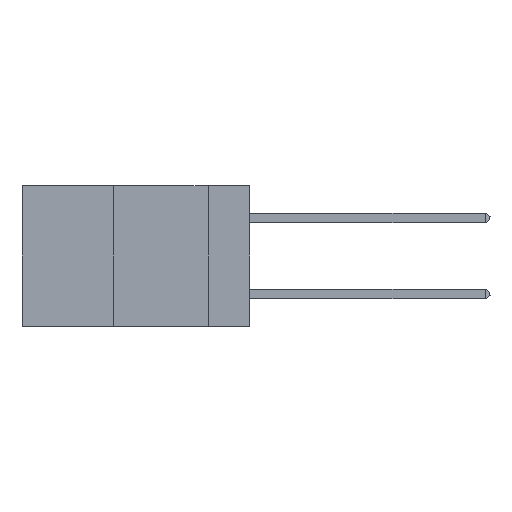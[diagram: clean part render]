
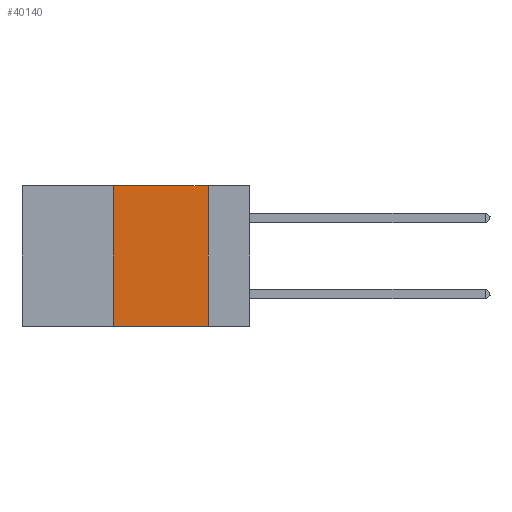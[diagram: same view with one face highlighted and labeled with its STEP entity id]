
A CAD part, left-side view. The second image highlights one B-rep face of the part: STEP entity #40140.
In plain terms, the highlighted planar face has unit normal (-1, 0, 0).
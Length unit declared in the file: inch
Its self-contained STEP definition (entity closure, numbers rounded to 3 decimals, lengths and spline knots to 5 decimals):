
#19 = LINE ( 'NONE', #12767, #11226 ) ;
#335 = EDGE_CURVE ( 'NONE', #4219, #24030, #37030, .T. ) ;
#2052 = ORIENTED_EDGE ( 'NONE', *, *, #5485, .F. ) ;
#3393 = VECTOR ( 'NONE', #3627, 39.37008 ) ;
#3627 = DIRECTION ( 'NONE',  ( 0., 0., 1. ) ) ;
#4219 = VERTEX_POINT ( 'NONE', #31498 ) ;
#5485 = EDGE_CURVE ( 'NONE', #18200, #18398, #17396, .T. ) ;
#7372 = ORIENTED_EDGE ( 'NONE', *, *, #30842, .F. ) ;
#7938 = EDGE_CURVE ( 'NONE', #4219, #18200, #34879, .T. ) ;
#9386 = ORIENTED_EDGE ( 'NONE', *, *, #7938, .F. ) ;
#11226 = VECTOR ( 'NONE', #29908, 39.37008 ) ;
#12767 = CARTESIAN_POINT ( 'NONE',  ( 0., 0.11, 0. ) ) ;
#14821 = CARTESIAN_POINT ( 'NONE',  ( 0., 0.11, -0.37 ) ) ;
#14947 = CARTESIAN_POINT ( 'NONE',  ( 0., 0.36, 0. ) ) ;
#16150 = CARTESIAN_POINT ( 'NONE',  ( 0., 0.6, 0. ) ) ;
#16752 = DIRECTION ( 'NONE',  ( 1., 0., 0. ) ) ;
#17072 = CARTESIAN_POINT ( 'NONE',  ( 0., 0.6, 0. ) ) ;
#17396 = LINE ( 'NONE', #17072, #42497 ) ;
#18200 = VERTEX_POINT ( 'NONE', #40072 ) ;
#18398 = VERTEX_POINT ( 'NONE', #37828 ) ;
#18749 = AXIS2_PLACEMENT_3D ( 'NONE', #16150, #16752, #44076 ) ;
#18891 = ORIENTED_EDGE ( 'NONE', *, *, #335, .T. ) ;
#23946 = DIRECTION ( 'NONE',  ( 0., -1., 0. ) ) ;
#24030 = VERTEX_POINT ( 'NONE', #14821 ) ;
#28546 = VECTOR ( 'NONE', #34064, 39.37008 ) ;
#29908 = DIRECTION ( 'NONE',  ( 0., 0., -1. ) ) ;
#30842 = EDGE_CURVE ( 'NONE', #18398, #24030, #19, .T. ) ;
#31498 = CARTESIAN_POINT ( 'NONE',  ( 0., 0.36, -0.37 ) ) ;
#32033 = FACE_OUTER_BOUND ( 'NONE', #39513, .T. ) ;
#34064 = DIRECTION ( 'NONE',  ( 0., -1., 0. ) ) ;
#34879 = LINE ( 'NONE', #14947, #3393 ) ;
#37030 = LINE ( 'NONE', #37489, #28546 ) ;
#37489 = CARTESIAN_POINT ( 'NONE',  ( 0., 0.6, -0.37 ) ) ;
#37828 = CARTESIAN_POINT ( 'NONE',  ( 0., 0.11, 0. ) ) ;
#39513 = EDGE_LOOP ( 'NONE', ( #7372, #2052, #9386, #18891 ) ) ;
#40072 = CARTESIAN_POINT ( 'NONE',  ( 0., 0.36, 0. ) ) ;
#40140 = ADVANCED_FACE ( 'NONE', ( #32033 ), #43774, .F. ) ;
#42497 = VECTOR ( 'NONE', #23946, 39.37008 ) ;
#43774 = PLANE ( 'NONE',  #18749 ) ;
#44076 = DIRECTION ( 'NONE',  ( 0., 0., -1. ) ) ;
